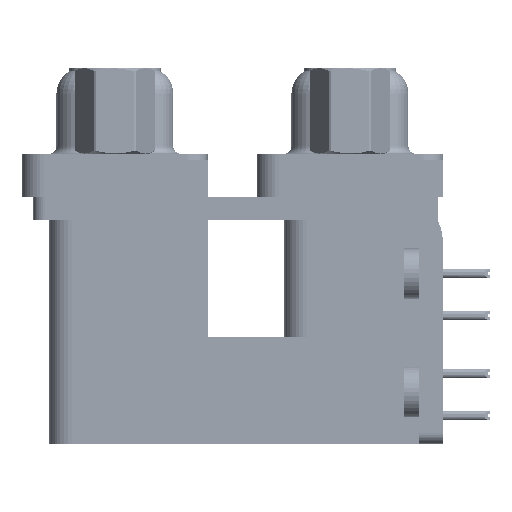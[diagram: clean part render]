
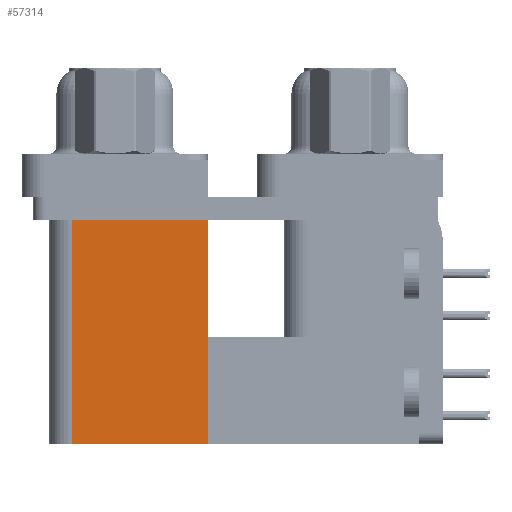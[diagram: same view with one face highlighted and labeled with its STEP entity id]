
A CAD part, left-side view. The second image highlights one B-rep face of the part: STEP entity #57314.
In plain terms, the highlighted planar face has unit normal (-1, 0, 0).
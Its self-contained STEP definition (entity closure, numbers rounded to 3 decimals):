
#562 = CARTESIAN_POINT ( 'NONE',  ( 3.7, 18.8, -19.2 ) ) ;
#2254 = FACE_OUTER_BOUND ( 'NONE', #54862, .T. ) ;
#5438 = AXIS2_PLACEMENT_3D ( 'NONE', #29647, #33436, #23145 ) ;
#10375 = CARTESIAN_POINT ( 'NONE',  ( 3.7, 9.6, -2.5 ) ) ;
#11609 = ORIENTED_EDGE ( 'NONE', *, *, #39443, .F. ) ;
#12194 = DIRECTION ( 'NONE',  ( 0., 0., 1. ) ) ;
#12428 = DIRECTION ( 'NONE',  ( 0., 0., 1. ) ) ;
#18129 = EDGE_CURVE ( 'NONE', #38782, #21029, #59382, .T. ) ;
#18239 = CARTESIAN_POINT ( 'NONE',  ( 3.7, 9.6, -19.2 ) ) ;
#19259 = CARTESIAN_POINT ( 'NONE',  ( 3.7, 18.8, -2.5 ) ) ;
#21029 = VERTEX_POINT ( 'NONE', #47339 ) ;
#23145 = DIRECTION ( 'NONE',  ( 0., 1., 0. ) ) ;
#24949 = EDGE_CURVE ( 'NONE', #21029, #48051, #32255, .T. ) ;
#25248 = CARTESIAN_POINT ( 'NONE',  ( 3.7, 9.6, -19.2 ) ) ;
#26766 = EDGE_CURVE ( 'NONE', #46193, #48051, #59136, .T. ) ;
#27724 = DIRECTION ( 'NONE',  ( 0., 1., 0. ) ) ;
#29647 = CARTESIAN_POINT ( 'NONE',  ( 3.7, 9.6, -19.2 ) ) ;
#32255 = LINE ( 'NONE', #10375, #59312 ) ;
#33436 = DIRECTION ( 'NONE',  ( 1., 0., 0. ) ) ;
#35224 = CARTESIAN_POINT ( 'NONE',  ( 3.7, 18.8, -19.2 ) ) ;
#37842 = ORIENTED_EDGE ( 'NONE', *, *, #24949, .T. ) ;
#38347 = CARTESIAN_POINT ( 'NONE',  ( 3.7, 9.6, -19.2 ) ) ;
#38782 = VERTEX_POINT ( 'NONE', #25248 ) ;
#39443 = EDGE_CURVE ( 'NONE', #38782, #46193, #53782, .T. ) ;
#40956 = ORIENTED_EDGE ( 'NONE', *, *, #26766, .F. ) ;
#45085 = PLANE ( 'NONE',  #5438 ) ;
#45214 = VECTOR ( 'NONE', #12194, 1000. ) ;
#45553 = VECTOR ( 'NONE', #12428, 1000. ) ;
#46193 = VERTEX_POINT ( 'NONE', #35224 ) ;
#47339 = CARTESIAN_POINT ( 'NONE',  ( 3.7, 9.6, -2.5 ) ) ;
#47708 = DIRECTION ( 'NONE',  ( 0., 1., 0. ) ) ;
#48051 = VERTEX_POINT ( 'NONE', #19259 ) ;
#53782 = LINE ( 'NONE', #38347, #63207 ) ;
#54862 = EDGE_LOOP ( 'NONE', ( #37842, #40956, #11609, #67631 ) ) ;
#57314 = ADVANCED_FACE ( 'NONE', ( #2254 ), #45085, .F. ) ;
#59136 = LINE ( 'NONE', #562, #45214 ) ;
#59312 = VECTOR ( 'NONE', #47708, 1000. ) ;
#59382 = LINE ( 'NONE', #18239, #45553 ) ;
#63207 = VECTOR ( 'NONE', #27724, 1000. ) ;
#67631 = ORIENTED_EDGE ( 'NONE', *, *, #18129, .T. ) ;
